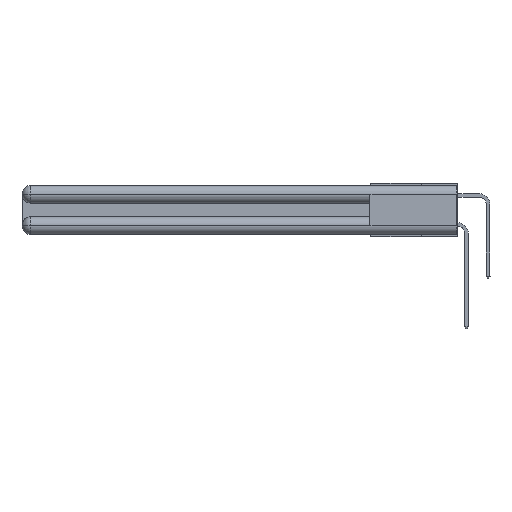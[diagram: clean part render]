
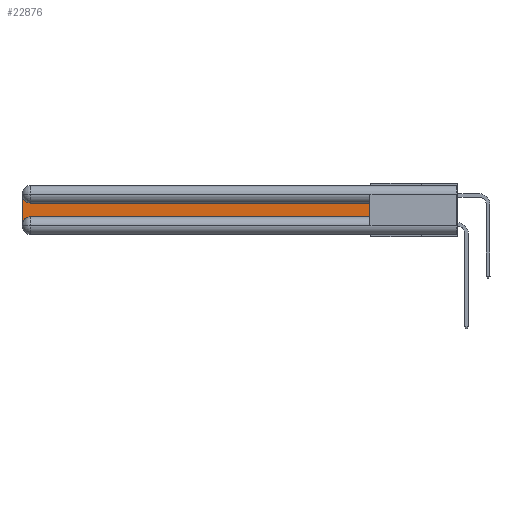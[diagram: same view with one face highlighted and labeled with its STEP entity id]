
A CAD part, left-side view. The second image highlights one B-rep face of the part: STEP entity #22876.
In plain terms, the highlighted planar face has unit normal (-1, 0, 0).
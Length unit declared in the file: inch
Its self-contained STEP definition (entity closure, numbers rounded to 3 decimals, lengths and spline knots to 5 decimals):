
#395 = VERTEX_POINT ( 'NONE', #17137 ) ;
#809 = DIRECTION ( 'NONE',  ( 1., 0., 0. ) ) ;
#1028 = DIRECTION ( 'NONE',  ( 0., 1., 0. ) ) ;
#1044 = CARTESIAN_POINT ( 'NONE',  ( 0.075, 3., -0.2175 ) ) ;
#3522 = LINE ( 'NONE', #19863, #28928 ) ;
#4113 = ORIENTED_EDGE ( 'NONE', *, *, #9472, .T. ) ;
#4796 = VERTEX_POINT ( 'NONE', #19333 ) ;
#8092 = ORIENTED_EDGE ( 'NONE', *, *, #27345, .T. ) ;
#8198 = CARTESIAN_POINT ( 'NONE',  ( 0.075, 2.94, -0.2175 ) ) ;
#9226 = DIRECTION ( 'NONE',  ( 0., 0., 1. ) ) ;
#9443 = ORIENTED_EDGE ( 'NONE', *, *, #25887, .T. ) ;
#9472 = EDGE_CURVE ( 'NONE', #10322, #395, #16510, .T. ) ;
#10092 = FACE_OUTER_BOUND ( 'NONE', #25866, .T. ) ;
#10121 = AXIS2_PLACEMENT_3D ( 'NONE', #14131, #809, #19554 ) ;
#10322 = VERTEX_POINT ( 'NONE', #15233 ) ;
#10828 = LINE ( 'NONE', #18768, #27421 ) ;
#12147 = DIRECTION ( 'NONE',  ( 0., -1., 0. ) ) ;
#12358 = VERTEX_POINT ( 'NONE', #13492 ) ;
#12904 = EDGE_CURVE ( 'NONE', #12358, #10322, #22388, .T. ) ;
#13492 = CARTESIAN_POINT ( 'NONE',  ( 0.075, 2.94, -0.1225 ) ) ;
#14031 = AXIS2_PLACEMENT_3D ( 'NONE', #23572, #25644, #28435 ) ;
#14131 = CARTESIAN_POINT ( 'NONE',  ( 0.075, 2.94, -0.2775 ) ) ;
#15233 = CARTESIAN_POINT ( 'NONE',  ( 0.075, 3., -0.0625 ) ) ;
#16236 = ORIENTED_EDGE ( 'NONE', *, *, #24271, .T. ) ;
#16510 = LINE ( 'NONE', #1044, #26884 ) ;
#16681 = VERTEX_POINT ( 'NONE', #8198 ) ;
#17137 = CARTESIAN_POINT ( 'NONE',  ( 0.075, 3., -0.2775 ) ) ;
#17316 = DIRECTION ( 'NONE',  ( 0., 0., -1. ) ) ;
#17333 = CIRCLE ( 'NONE', #10121, 0.06 ) ;
#18726 = PLANE ( 'NONE',  #14031 ) ;
#18768 = CARTESIAN_POINT ( 'NONE',  ( 0.075, 0.6, -0.2175 ) ) ;
#19333 = CARTESIAN_POINT ( 'NONE',  ( 0.075, 0.6, -0.1225 ) ) ;
#19554 = DIRECTION ( 'NONE',  ( 0., 0., -1. ) ) ;
#19863 = CARTESIAN_POINT ( 'NONE',  ( 0.075, 0.6, -0.1225 ) ) ;
#20719 = EDGE_CURVE ( 'NONE', #4796, #12358, #3522, .T. ) ;
#22388 = CIRCLE ( 'NONE', #28492, 0.06 ) ;
#22876 = ADVANCED_FACE ( 'NONE', ( #10092 ), #18726, .F. ) ;
#23572 = CARTESIAN_POINT ( 'NONE',  ( 0.075, 3., -0.1225 ) ) ;
#24102 = CARTESIAN_POINT ( 'NONE',  ( 0.075, 0.6, -0.2175 ) ) ;
#24134 = ORIENTED_EDGE ( 'NONE', *, *, #12904, .T. ) ;
#24271 = EDGE_CURVE ( 'NONE', #395, #16681, #17333, .T. ) ;
#25118 = CARTESIAN_POINT ( 'NONE',  ( 0.075, 2.94, -0.0625 ) ) ;
#25644 = DIRECTION ( 'NONE',  ( 1., 0., 0. ) ) ;
#25866 = EDGE_LOOP ( 'NONE', ( #27718, #24134, #4113, #16236, #9443, #8092 ) ) ;
#25887 = EDGE_CURVE ( 'NONE', #16681, #26307, #29004, .T. ) ;
#26307 = VERTEX_POINT ( 'NONE', #26342 ) ;
#26342 = CARTESIAN_POINT ( 'NONE',  ( 0.075, 0.6, -0.2175 ) ) ;
#26884 = VECTOR ( 'NONE', #17316, 39.37008 ) ;
#27297 = DIRECTION ( 'NONE',  ( 0., 0., -1. ) ) ;
#27345 = EDGE_CURVE ( 'NONE', #26307, #4796, #10828, .T. ) ;
#27421 = VECTOR ( 'NONE', #9226, 39.37008 ) ;
#27718 = ORIENTED_EDGE ( 'NONE', *, *, #20719, .T. ) ;
#28435 = DIRECTION ( 'NONE',  ( 0., 0., -1. ) ) ;
#28492 = AXIS2_PLACEMENT_3D ( 'NONE', #25118, #29879, #27297 ) ;
#28928 = VECTOR ( 'NONE', #1028, 39.37008 ) ;
#29004 = LINE ( 'NONE', #24102, #30480 ) ;
#29879 = DIRECTION ( 'NONE',  ( 1., 0., 0. ) ) ;
#30480 = VECTOR ( 'NONE', #12147, 39.37008 ) ;
